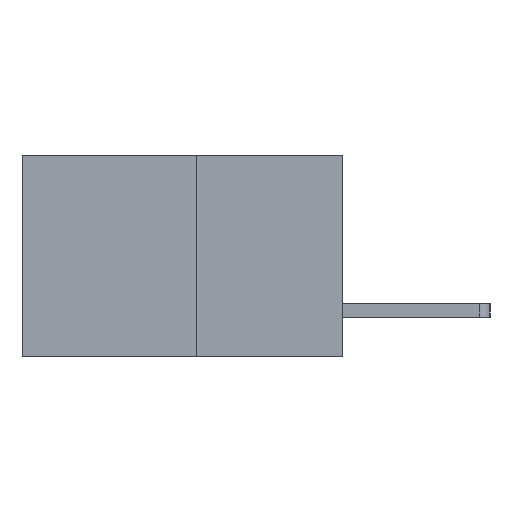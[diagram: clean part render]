
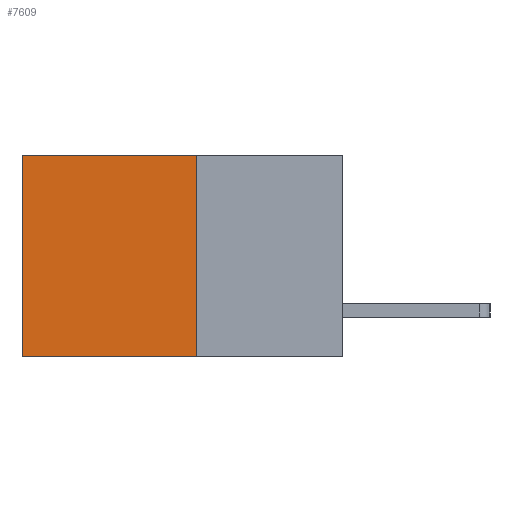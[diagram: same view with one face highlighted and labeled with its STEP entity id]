
A CAD part, left-side view. The second image highlights one B-rep face of the part: STEP entity #7609.
In plain terms, the highlighted planar face has unit normal (-1, 0, 0).
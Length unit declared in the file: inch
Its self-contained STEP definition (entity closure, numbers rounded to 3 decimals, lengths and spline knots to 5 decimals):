
#16 = CARTESIAN_POINT ( 'NONE',  ( 0.277, 0.59, -0.37 ) ) ;
#166 = CARTESIAN_POINT ( 'NONE',  ( 0.277, 0.27, -0.37 ) ) ;
#182 = EDGE_CURVE ( 'NONE', #1926, #7735, #4228, .T. ) ;
#505 = DIRECTION ( 'NONE',  ( 1., 0., 0. ) ) ;
#634 = DIRECTION ( 'NONE',  ( 0., 0., -1. ) ) ;
#744 = EDGE_CURVE ( 'NONE', #2104, #7735, #3224, .T. ) ;
#989 = PLANE ( 'NONE',  #9656 ) ;
#1826 = EDGE_CURVE ( 'NONE', #4463, #2104, #8166, .T. ) ;
#1876 = ORIENTED_EDGE ( 'NONE', *, *, #744, .T. ) ;
#1926 = VERTEX_POINT ( 'NONE', #5935 ) ;
#2104 = VERTEX_POINT ( 'NONE', #4527 ) ;
#2353 = LINE ( 'NONE', #5059, #4244 ) ;
#2500 = ORIENTED_EDGE ( 'NONE', *, *, #4356, .F. ) ;
#2914 = CARTESIAN_POINT ( 'NONE',  ( 0.277, 0.27, 0. ) ) ;
#3224 = LINE ( 'NONE', #5463, #7012 ) ;
#3294 = FACE_OUTER_BOUND ( 'NONE', #5097, .T. ) ;
#3499 = ORIENTED_EDGE ( 'NONE', *, *, #1826, .T. ) ;
#3954 = VECTOR ( 'NONE', #8110, 39.37008 ) ;
#4228 = LINE ( 'NONE', #9307, #7498 ) ;
#4244 = VECTOR ( 'NONE', #8072, 39.37008 ) ;
#4356 = EDGE_CURVE ( 'NONE', #4463, #1926, #2353, .T. ) ;
#4463 = VERTEX_POINT ( 'NONE', #2914 ) ;
#4527 = CARTESIAN_POINT ( 'NONE',  ( 0.277, 0.59, 0. ) ) ;
#5059 = CARTESIAN_POINT ( 'NONE',  ( 0.277, 0.27, -0.37 ) ) ;
#5097 = EDGE_LOOP ( 'NONE', ( #1876, #5334, #2500, #3499 ) ) ;
#5334 = ORIENTED_EDGE ( 'NONE', *, *, #182, .F. ) ;
#5463 = CARTESIAN_POINT ( 'NONE',  ( 0.277, 0.59, -0.37 ) ) ;
#5935 = CARTESIAN_POINT ( 'NONE',  ( 0.277, 0.27, -0.37 ) ) ;
#6753 = DIRECTION ( 'NONE',  ( 0., 1., 0. ) ) ;
#7012 = VECTOR ( 'NONE', #9633, 39.37008 ) ;
#7444 = CARTESIAN_POINT ( 'NONE',  ( 0.277, 0.27, 0. ) ) ;
#7498 = VECTOR ( 'NONE', #6753, 39.37008 ) ;
#7609 = ADVANCED_FACE ( 'NONE', ( #3294 ), #989, .F. ) ;
#7735 = VERTEX_POINT ( 'NONE', #16 ) ;
#8072 = DIRECTION ( 'NONE',  ( 0., 0., -1. ) ) ;
#8110 = DIRECTION ( 'NONE',  ( 0., 1., 0. ) ) ;
#8166 = LINE ( 'NONE', #7444, #3954 ) ;
#9307 = CARTESIAN_POINT ( 'NONE',  ( 0.277, 0.27, -0.37 ) ) ;
#9633 = DIRECTION ( 'NONE',  ( 0., 0., -1. ) ) ;
#9656 = AXIS2_PLACEMENT_3D ( 'NONE', #166, #505, #634 ) ;
